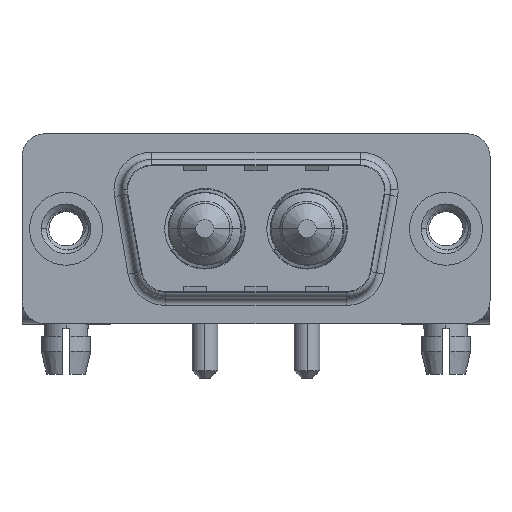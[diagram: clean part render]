
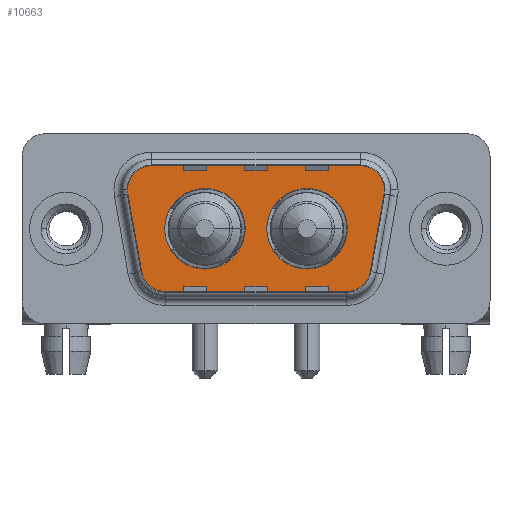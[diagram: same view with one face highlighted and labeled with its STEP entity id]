
A CAD part, top view. The second image highlights one B-rep face of the part: STEP entity #10663.
In plain terms, the highlighted planar face has unit normal (0, 0, 1).
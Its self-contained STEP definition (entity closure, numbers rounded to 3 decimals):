
#70 = DIRECTION ( 'NONE',  ( 1., 0., 0. ) ) ;
#94 = ORIENTED_EDGE ( 'NONE', *, *, #7949, .T. ) ;
#213 = VECTOR ( 'NONE', #12362, 1000. ) ;
#443 = CIRCLE ( 'NONE', #10017, 2. ) ;
#465 = VERTEX_POINT ( 'NONE', #11773 ) ;
#492 = CIRCLE ( 'NONE', #9620, 2.65 ) ;
#551 = DIRECTION ( 'NONE',  ( 1., 0., 0. ) ) ;
#690 = CIRCLE ( 'NONE', #9597, 2. ) ;
#811 = CARTESIAN_POINT ( 'NONE',  ( 19.564, 2.9, 0. ) ) ;
#827 = DIRECTION ( 'NONE',  ( 1., 0., 0. ) ) ;
#833 = CIRCLE ( 'NONE', #2887, 2. ) ;
#906 = CARTESIAN_POINT ( 'NONE',  ( 21.534, 2.553, 0. ) ) ;
#948 = CARTESIAN_POINT ( 'NONE',  ( 9.14, 0., 0. ) ) ;
#1064 = DIRECTION ( 'NONE',  ( -1., 0., 0. ) ) ;
#1271 = DIRECTION ( 'NONE',  ( 0., 0., 1. ) ) ;
#1694 = EDGE_CURVE ( 'NONE', #13262, #11944, #690, .T. ) ;
#1701 = CIRCLE ( 'NONE', #11274, 2. ) ;
#2250 = EDGE_CURVE ( 'NONE', #10928, #4744, #13279, .T. ) ;
#2269 = CARTESIAN_POINT ( 'NONE',  ( 5.436, 4.9, 0. ) ) ;
#2494 = LINE ( 'NONE', #13435, #12490 ) ;
#2509 = DIRECTION ( 'NONE',  ( 0., 0., 1. ) ) ;
#2534 = EDGE_CURVE ( 'NONE', #4366, #7619, #12006, .T. ) ;
#2713 = AXIS2_PLACEMENT_3D ( 'NONE', #10551, #12841, #9486 ) ;
#2776 = DIRECTION ( 'NONE',  ( 0., 0., 1. ) ) ;
#2887 = AXIS2_PLACEMENT_3D ( 'NONE', #10860, #1271, #1064 ) ;
#3103 = ORIENTED_EDGE ( 'NONE', *, *, #12337, .T. ) ;
#3131 = PLANE ( 'NONE',  #6314 ) ;
#3228 = AXIS2_PLACEMENT_3D ( 'NONE', #811, #13686, #10465 ) ;
#3401 = CARTESIAN_POINT ( 'NONE',  ( 11.79, 0., 0. ) ) ;
#3630 = CARTESIAN_POINT ( 'NONE',  ( 5.436, 4.9, 0. ) ) ;
#3677 = CARTESIAN_POINT ( 'NONE',  ( 3.466, 2.553, 0. ) ) ;
#3694 = ORIENTED_EDGE ( 'NONE', *, *, #1694, .T. ) ;
#3819 = EDGE_CURVE ( 'NONE', #13839, #7080, #492, .T. ) ;
#3906 = ORIENTED_EDGE ( 'NONE', *, *, #6737, .T. ) ;
#4073 = CARTESIAN_POINT ( 'NONE',  ( 4.489, -3.247, 0. ) ) ;
#4083 = ORIENTED_EDGE ( 'NONE', *, *, #2534, .F. ) ;
#4159 = VERTEX_POINT ( 'NONE', #4073 ) ;
#4264 = DIRECTION ( 'NONE',  ( 1., 0., 0. ) ) ;
#4366 = VERTEX_POINT ( 'NONE', #3401 ) ;
#4726 = CARTESIAN_POINT ( 'NONE',  ( 18.541, -4.9, 0. ) ) ;
#4744 = VERTEX_POINT ( 'NONE', #10698 ) ;
#5064 = CARTESIAN_POINT ( 'NONE',  ( 20.511, -3.247, 0. ) ) ;
#5149 = ORIENTED_EDGE ( 'NONE', *, *, #10759, .T. ) ;
#5253 = DIRECTION ( 'NONE',  ( 0.174, 0.985, 0. ) ) ;
#5445 = CIRCLE ( 'NONE', #2713, 2.65 ) ;
#5469 = CARTESIAN_POINT ( 'NONE',  ( 18.51, 0., 0. ) ) ;
#5491 = DIRECTION ( 'NONE',  ( 0., 0., 1. ) ) ;
#5622 = FACE_OUTER_BOUND ( 'NONE', #13412, .T. ) ;
#5945 = LINE ( 'NONE', #12390, #8375 ) ;
#6216 = EDGE_CURVE ( 'NONE', #7080, #13839, #5445, .T. ) ;
#6260 = DIRECTION ( 'NONE',  ( 0., 0., 1. ) ) ;
#6291 = EDGE_CURVE ( 'NONE', #11944, #10928, #10699, .T. ) ;
#6314 = AXIS2_PLACEMENT_3D ( 'NONE', #6635, #14132, #4264 ) ;
#6392 = ORIENTED_EDGE ( 'NONE', *, *, #11904, .F. ) ;
#6530 = ORIENTED_EDGE ( 'NONE', *, *, #6655, .T. ) ;
#6635 = CARTESIAN_POINT ( 'NONE',  ( 18.541, -2.9, 0. ) ) ;
#6655 = EDGE_CURVE ( 'NONE', #8285, #7025, #12505, .T. ) ;
#6737 = EDGE_CURVE ( 'NONE', #4744, #8285, #443, .T. ) ;
#7012 = DIRECTION ( 'NONE',  ( 1., 0., 0. ) ) ;
#7025 = VERTEX_POINT ( 'NONE', #2269 ) ;
#7067 = DIRECTION ( 'NONE',  ( 1., 0., 0. ) ) ;
#7080 = VERTEX_POINT ( 'NONE', #5469 ) ;
#7333 = CARTESIAN_POINT ( 'NONE',  ( 15.86, 0., 0. ) ) ;
#7557 = CARTESIAN_POINT ( 'NONE',  ( 19.564, 4.9, 0. ) ) ;
#7619 = VERTEX_POINT ( 'NONE', #10316 ) ;
#7775 = ORIENTED_EDGE ( 'NONE', *, *, #6216, .F. ) ;
#7858 = CARTESIAN_POINT ( 'NONE',  ( 5.436, 2.9, 0. ) ) ;
#7949 = EDGE_CURVE ( 'NONE', #7025, #8559, #1701, .T. ) ;
#7960 = VECTOR ( 'NONE', #5253, 1000. ) ;
#8055 = CARTESIAN_POINT ( 'NONE',  ( 21.534, 2.553, 0. ) ) ;
#8119 = CARTESIAN_POINT ( 'NONE',  ( 18.541, -2.9, 0. ) ) ;
#8285 = VERTEX_POINT ( 'NONE', #7557 ) ;
#8375 = VECTOR ( 'NONE', #13465, 1000. ) ;
#8559 = VERTEX_POINT ( 'NONE', #3677 ) ;
#8626 = FACE_BOUND ( 'NONE', #10572, .T. ) ;
#8797 = AXIS2_PLACEMENT_3D ( 'NONE', #948, #12170, #9085 ) ;
#9085 = DIRECTION ( 'NONE',  ( 1., 0., 0. ) ) ;
#9134 = CARTESIAN_POINT ( 'NONE',  ( 19.564, 2.9, 0. ) ) ;
#9434 = EDGE_LOOP ( 'NONE', ( #7775, #13236 ) ) ;
#9486 = DIRECTION ( 'NONE',  ( 1., 0., 0. ) ) ;
#9597 = AXIS2_PLACEMENT_3D ( 'NONE', #8119, #5491, #551 ) ;
#9620 = AXIS2_PLACEMENT_3D ( 'NONE', #7333, #6260, #827 ) ;
#9716 = ORIENTED_EDGE ( 'NONE', *, *, #11293, .T. ) ;
#9860 = DIRECTION ( 'NONE',  ( 0., 0., 1. ) ) ;
#10017 = AXIS2_PLACEMENT_3D ( 'NONE', #9134, #2776, #11500 ) ;
#10316 = CARTESIAN_POINT ( 'NONE',  ( 6.49, 0., 0. ) ) ;
#10459 = CIRCLE ( 'NONE', #14100, 2.65 ) ;
#10465 = DIRECTION ( 'NONE',  ( -1., 0., 0. ) ) ;
#10551 = CARTESIAN_POINT ( 'NONE',  ( 15.86, 0., 0. ) ) ;
#10572 = EDGE_LOOP ( 'NONE', ( #4083, #6392 ) ) ;
#10663 = ADVANCED_FACE ( 'NONE', ( #13065, #8626, #5622 ), #3131, .T. ) ;
#10698 = CARTESIAN_POINT ( 'NONE',  ( 21.564, 2.9, 0. ) ) ;
#10699 = LINE ( 'NONE', #906, #7960 ) ;
#10759 = EDGE_CURVE ( 'NONE', #4159, #465, #833, .T. ) ;
#10860 = CARTESIAN_POINT ( 'NONE',  ( 6.459, -2.9, 0. ) ) ;
#10928 = VERTEX_POINT ( 'NONE', #8055 ) ;
#11274 = AXIS2_PLACEMENT_3D ( 'NONE', #7858, #9860, #70 ) ;
#11293 = EDGE_CURVE ( 'NONE', #8559, #4159, #5945, .T. ) ;
#11322 = ORIENTED_EDGE ( 'NONE', *, *, #2250, .T. ) ;
#11500 = DIRECTION ( 'NONE',  ( -1., 0., 0. ) ) ;
#11773 = CARTESIAN_POINT ( 'NONE',  ( 6.459, -4.9, 0. ) ) ;
#11904 = EDGE_CURVE ( 'NONE', #7619, #4366, #10459, .T. ) ;
#11944 = VERTEX_POINT ( 'NONE', #5064 ) ;
#12006 = CIRCLE ( 'NONE', #8797, 2.65 ) ;
#12170 = DIRECTION ( 'NONE',  ( 0., 0., 1. ) ) ;
#12307 = CARTESIAN_POINT ( 'NONE',  ( 9.14, 0., 0. ) ) ;
#12337 = EDGE_CURVE ( 'NONE', #465, #13262, #2494, .T. ) ;
#12362 = DIRECTION ( 'NONE',  ( -1., 0., 0. ) ) ;
#12390 = CARTESIAN_POINT ( 'NONE',  ( 3.466, 2.553, 0. ) ) ;
#12490 = VECTOR ( 'NONE', #7067, 1000. ) ;
#12505 = LINE ( 'NONE', #3630, #213 ) ;
#12673 = ORIENTED_EDGE ( 'NONE', *, *, #6291, .T. ) ;
#12841 = DIRECTION ( 'NONE',  ( 0., 0., 1. ) ) ;
#13065 = FACE_BOUND ( 'NONE', #9434, .T. ) ;
#13236 = ORIENTED_EDGE ( 'NONE', *, *, #3819, .F. ) ;
#13262 = VERTEX_POINT ( 'NONE', #4726 ) ;
#13279 = CIRCLE ( 'NONE', #3228, 2. ) ;
#13286 = CARTESIAN_POINT ( 'NONE',  ( 13.21, 0., 0. ) ) ;
#13412 = EDGE_LOOP ( 'NONE', ( #3694, #12673, #11322, #3906, #6530, #94, #9716, #5149, #3103 ) ) ;
#13435 = CARTESIAN_POINT ( 'NONE',  ( 6.459, -4.9, 0. ) ) ;
#13465 = DIRECTION ( 'NONE',  ( 0.174, -0.985, 0. ) ) ;
#13686 = DIRECTION ( 'NONE',  ( 0., 0., 1. ) ) ;
#13839 = VERTEX_POINT ( 'NONE', #13286 ) ;
#14100 = AXIS2_PLACEMENT_3D ( 'NONE', #12307, #2509, #7012 ) ;
#14132 = DIRECTION ( 'NONE',  ( 0., 0., 1. ) ) ;
